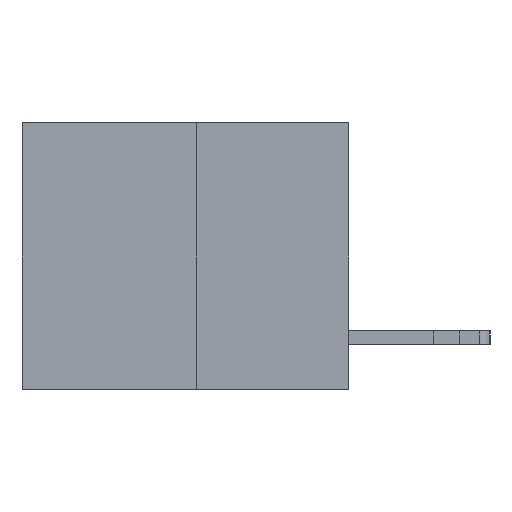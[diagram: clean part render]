
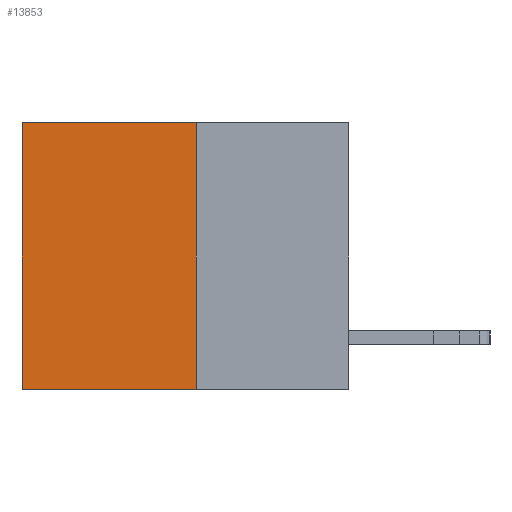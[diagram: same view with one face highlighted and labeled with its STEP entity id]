
A CAD part, left-side view. The second image highlights one B-rep face of the part: STEP entity #13853.
In plain terms, the highlighted planar face has unit normal (-1, 0, 0).
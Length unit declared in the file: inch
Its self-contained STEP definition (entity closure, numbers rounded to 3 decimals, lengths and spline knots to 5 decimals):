
#540 = VERTEX_POINT ( 'NONE', #12477 ) ;
#2670 = ORIENTED_EDGE ( 'NONE', *, *, #19124, .T. ) ;
#2920 = EDGE_CURVE ( 'NONE', #540, #3531, #14977, .T. ) ;
#3505 = LINE ( 'NONE', #23094, #22256 ) ;
#3531 = VERTEX_POINT ( 'NONE', #17698 ) ;
#4342 = DIRECTION ( 'NONE',  ( 1., 0., 0. ) ) ;
#4893 = CARTESIAN_POINT ( 'NONE',  ( 0.3165, 0.28, -0.49 ) ) ;
#4899 = VERTEX_POINT ( 'NONE', #14044 ) ;
#6411 = EDGE_CURVE ( 'NONE', #7533, #540, #18717, .T. ) ;
#7533 = VERTEX_POINT ( 'NONE', #7931 ) ;
#7931 = CARTESIAN_POINT ( 'NONE',  ( 0.3165, 0.28, 0. ) ) ;
#8354 = DIRECTION ( 'NONE',  ( 0., 1., 0. ) ) ;
#10776 = CARTESIAN_POINT ( 'NONE',  ( 0.3165, 0.28, -0.49 ) ) ;
#12364 = DIRECTION ( 'NONE',  ( 0., 0., -1. ) ) ;
#12477 = CARTESIAN_POINT ( 'NONE',  ( 0.3165, 0.28, -0.49 ) ) ;
#12635 = DIRECTION ( 'NONE',  ( 0., 1., 0. ) ) ;
#12818 = VECTOR ( 'NONE', #18787, 39.37008 ) ;
#12873 = AXIS2_PLACEMENT_3D ( 'NONE', #14844, #4342, #16558 ) ;
#13680 = CARTESIAN_POINT ( 'NONE',  ( 0.3165, 0.28, 0. ) ) ;
#13748 = ORIENTED_EDGE ( 'NONE', *, *, #2920, .F. ) ;
#13853 = ADVANCED_FACE ( 'NONE', ( #20342 ), #18621, .F. ) ;
#14044 = CARTESIAN_POINT ( 'NONE',  ( 0.3165, 0.6, 0. ) ) ;
#14844 = CARTESIAN_POINT ( 'NONE',  ( 0.3165, 0.28, -0.49 ) ) ;
#14941 = LINE ( 'NONE', #13680, #19163 ) ;
#14977 = LINE ( 'NONE', #10776, #18049 ) ;
#15130 = EDGE_LOOP ( 'NONE', ( #19795, #13748, #17432, #2670 ) ) ;
#16558 = DIRECTION ( 'NONE',  ( 0., 0., -1. ) ) ;
#17432 = ORIENTED_EDGE ( 'NONE', *, *, #6411, .F. ) ;
#17698 = CARTESIAN_POINT ( 'NONE',  ( 0.3165, 0.6, -0.49 ) ) ;
#18049 = VECTOR ( 'NONE', #12635, 39.37008 ) ;
#18609 = EDGE_CURVE ( 'NONE', #4899, #3531, #3505, .T. ) ;
#18621 = PLANE ( 'NONE',  #12873 ) ;
#18717 = LINE ( 'NONE', #4893, #12818 ) ;
#18787 = DIRECTION ( 'NONE',  ( 0., 0., -1. ) ) ;
#19124 = EDGE_CURVE ( 'NONE', #7533, #4899, #14941, .T. ) ;
#19163 = VECTOR ( 'NONE', #8354, 39.37008 ) ;
#19795 = ORIENTED_EDGE ( 'NONE', *, *, #18609, .T. ) ;
#20342 = FACE_OUTER_BOUND ( 'NONE', #15130, .T. ) ;
#22256 = VECTOR ( 'NONE', #12364, 39.37008 ) ;
#23094 = CARTESIAN_POINT ( 'NONE',  ( 0.3165, 0.6, -0.49 ) ) ;
